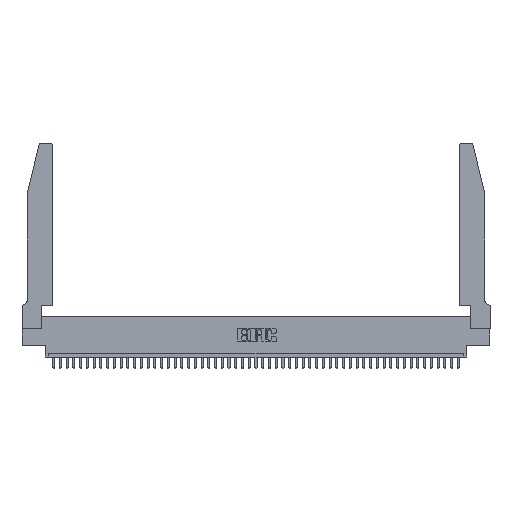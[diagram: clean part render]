
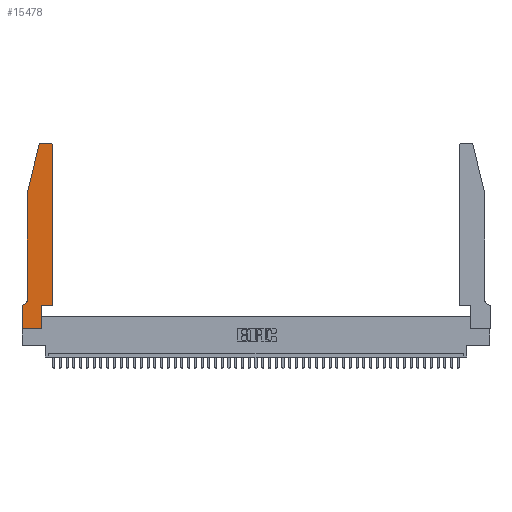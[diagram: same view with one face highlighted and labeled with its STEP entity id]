
A CAD part, top view. The second image highlights one B-rep face of the part: STEP entity #15478.
In plain terms, the highlighted planar face has unit normal (0, 0, 1).
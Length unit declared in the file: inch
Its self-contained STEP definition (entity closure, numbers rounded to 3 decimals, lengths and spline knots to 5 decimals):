
#88 = ORIENTED_EDGE ( 'NONE', *, *, #6962, .T. ) ;
#566 = CARTESIAN_POINT ( 'NONE',  ( 0., 0.35, 0.37 ) ) ;
#2548 = LINE ( 'NONE', #25278, #21240 ) ;
#2720 = DIRECTION ( 'NONE',  ( 0., 1., 0. ) ) ;
#3032 = VERTEX_POINT ( 'NONE', #42232 ) ;
#3805 = AXIS2_PLACEMENT_3D ( 'NONE', #36705, #41069, #40446 ) ;
#4126 = LINE ( 'NONE', #10552, #36232 ) ;
#6044 = VECTOR ( 'NONE', #23524, 39.37008 ) ;
#6074 = VERTEX_POINT ( 'NONE', #7845 ) ;
#6962 = EDGE_CURVE ( 'NONE', #32405, #3032, #40189, .T. ) ;
#7144 = CARTESIAN_POINT ( 'NONE',  ( 0.0055, 0.42, 0.37 ) ) ;
#7160 = EDGE_CURVE ( 'NONE', #43661, #17790, #11598, .T. ) ;
#7193 = LINE ( 'NONE', #15904, #6044 ) ;
#7311 = CARTESIAN_POINT ( 'NONE',  ( 0.2605, 2.75, 0.37 ) ) ;
#7845 = CARTESIAN_POINT ( 'NONE',  ( 0.2865, 0., 0.37 ) ) ;
#8034 = CIRCLE ( 'NONE', #22942, 0.03 ) ;
#9310 = DIRECTION ( 'NONE',  ( -1., 0., 0. ) ) ;
#9410 = VECTOR ( 'NONE', #21468, 39.37008 ) ;
#9710 = CARTESIAN_POINT ( 'NONE',  ( 0., 0.35, 0.37 ) ) ;
#10404 = ORIENTED_EDGE ( 'NONE', *, *, #36614, .T. ) ;
#10552 = CARTESIAN_POINT ( 'NONE',  ( 0.0755, 2., 0.37 ) ) ;
#10879 = DIRECTION ( 'NONE',  ( -1., 0., 0. ) ) ;
#11598 = LINE ( 'NONE', #15957, #30310 ) ;
#11695 = CIRCLE ( 'NONE', #18827, 0.07 ) ;
#13011 = EDGE_CURVE ( 'NONE', #21215, #30561, #38854, .T. ) ;
#13251 = LINE ( 'NONE', #7311, #25518 ) ;
#14350 = DIRECTION ( 'NONE',  ( 0., 0., -1. ) ) ;
#14723 = VERTEX_POINT ( 'NONE', #16777 ) ;
#14812 = VERTEX_POINT ( 'NONE', #39039 ) ;
#15478 = ADVANCED_FACE ( 'NONE', ( #28745 ), #26694, .T. ) ;
#15545 = CARTESIAN_POINT ( 'NONE',  ( 0., 0., 0.37 ) ) ;
#15624 = VECTOR ( 'NONE', #9310, 39.37008 ) ;
#15684 = ORIENTED_EDGE ( 'NONE', *, *, #27631, .T. ) ;
#15904 = CARTESIAN_POINT ( 'NONE',  ( 0., 0., 0.37 ) ) ;
#15957 = CARTESIAN_POINT ( 'NONE',  ( 0.4505, 0.35, 0.37 ) ) ;
#16777 = CARTESIAN_POINT ( 'NONE',  ( 0.284, 2.75, 0.37 ) ) ;
#17431 = CARTESIAN_POINT ( 'NONE',  ( 0.4505, 0.35, 0.37 ) ) ;
#17790 = VERTEX_POINT ( 'NONE', #17431 ) ;
#18008 = DIRECTION ( 'NONE',  ( 0., 0., 1. ) ) ;
#18670 = ORIENTED_EDGE ( 'NONE', *, *, #43840, .T. ) ;
#18827 = AXIS2_PLACEMENT_3D ( 'NONE', #7144, #14350, #10879 ) ;
#19296 = LINE ( 'NONE', #43368, #9410 ) ;
#19602 = ORIENTED_EDGE ( 'NONE', *, *, #7160, .T. ) ;
#20277 = VERTEX_POINT ( 'NONE', #28497 ) ;
#20311 = VECTOR ( 'NONE', #39492, 39.37008 ) ;
#21215 = VERTEX_POINT ( 'NONE', #9710 ) ;
#21240 = VECTOR ( 'NONE', #2720, 39.37008 ) ;
#21468 = DIRECTION ( 'NONE',  ( 0., 1., 0. ) ) ;
#21823 = ORIENTED_EDGE ( 'NONE', *, *, #35399, .T. ) ;
#21848 = ORIENTED_EDGE ( 'NONE', *, *, #22496, .T. ) ;
#22496 = EDGE_CURVE ( 'NONE', #6074, #43661, #19296, .T. ) ;
#22669 = ORIENTED_EDGE ( 'NONE', *, *, #40608, .T. ) ;
#22921 = DIRECTION ( 'NONE',  ( 1., 0., 0. ) ) ;
#22942 = AXIS2_PLACEMENT_3D ( 'NONE', #32560, #18008, #44121 ) ;
#23524 = DIRECTION ( 'NONE',  ( 1., 0., 0. ) ) ;
#24866 = CARTESIAN_POINT ( 'NONE',  ( 0.0755, 0.42, 0.37 ) ) ;
#25278 = CARTESIAN_POINT ( 'NONE',  ( 0.4505, 0.35, 0.37 ) ) ;
#25518 = VECTOR ( 'NONE', #44655, 39.37008 ) ;
#25780 = VERTEX_POINT ( 'NONE', #24866 ) ;
#26415 = ORIENTED_EDGE ( 'NONE', *, *, #13011, .T. ) ;
#26441 = CARTESIAN_POINT ( 'NONE',  ( 0.0055, 0.35, 0.37 ) ) ;
#26443 = DIRECTION ( 'NONE',  ( 0., -1., 0. ) ) ;
#26694 = PLANE ( 'NONE',  #39971 ) ;
#27224 = ORIENTED_EDGE ( 'NONE', *, *, #38644, .T. ) ;
#27432 = CARTESIAN_POINT ( 'NONE',  ( 0.0755, 0.35, 0.37 ) ) ;
#27631 = EDGE_CURVE ( 'NONE', #25780, #32143, #11695, .T. ) ;
#28424 = CARTESIAN_POINT ( 'NONE',  ( 0.25487, 2.72718, 0.37 ) ) ;
#28497 = CARTESIAN_POINT ( 'NONE',  ( 0.4505, 2.72, 0.37 ) ) ;
#28745 = FACE_OUTER_BOUND ( 'NONE', #44718, .T. ) ;
#30133 = DIRECTION ( 'NONE',  ( 1., 0., 0. ) ) ;
#30310 = VECTOR ( 'NONE', #22921, 39.37008 ) ;
#30561 = VERTEX_POINT ( 'NONE', #37762 ) ;
#30996 = EDGE_CURVE ( 'NONE', #20277, #14812, #8034, .T. ) ;
#31943 = CIRCLE ( 'NONE', #3805, 0.03 ) ;
#32143 = VERTEX_POINT ( 'NONE', #26441 ) ;
#32405 = VERTEX_POINT ( 'NONE', #28424 ) ;
#32560 = CARTESIAN_POINT ( 'NONE',  ( 0.4205, 2.72, 0.37 ) ) ;
#34161 = VECTOR ( 'NONE', #26443, 39.37008 ) ;
#35399 = EDGE_CURVE ( 'NONE', #32143, #21215, #35485, .T. ) ;
#35485 = LINE ( 'NONE', #27432, #15624 ) ;
#35905 = CARTESIAN_POINT ( 'NONE',  ( 0.0755, 2., 0.37 ) ) ;
#36232 = VECTOR ( 'NONE', #48362, 39.37008 ) ;
#36260 = ORIENTED_EDGE ( 'NONE', *, *, #30996, .T. ) ;
#36614 = EDGE_CURVE ( 'NONE', #17790, #20277, #2548, .T. ) ;
#36705 = CARTESIAN_POINT ( 'NONE',  ( 0.284, 2.72, 0.37 ) ) ;
#37762 = CARTESIAN_POINT ( 'NONE',  ( 0., 0., 0.37 ) ) ;
#38644 = EDGE_CURVE ( 'NONE', #3032, #25780, #4126, .T. ) ;
#38854 = LINE ( 'NONE', #15545, #34161 ) ;
#39039 = CARTESIAN_POINT ( 'NONE',  ( 0.4205, 2.75, 0.37 ) ) ;
#39492 = DIRECTION ( 'NONE',  ( -0.239, -0.971, 0. ) ) ;
#39971 = AXIS2_PLACEMENT_3D ( 'NONE', #566, #41860, #30133 ) ;
#40189 = LINE ( 'NONE', #35905, #20311 ) ;
#40446 = DIRECTION ( 'NONE',  ( 1., 0., 0. ) ) ;
#40608 = EDGE_CURVE ( 'NONE', #30561, #6074, #7193, .T. ) ;
#41069 = DIRECTION ( 'NONE',  ( 0., 0., 1. ) ) ;
#41860 = DIRECTION ( 'NONE',  ( 0., 0., 1. ) ) ;
#42232 = CARTESIAN_POINT ( 'NONE',  ( 0.0755, 2., 0.37 ) ) ;
#43368 = CARTESIAN_POINT ( 'NONE',  ( 0.2865, 0.35, 0.37 ) ) ;
#43661 = VERTEX_POINT ( 'NONE', #43723 ) ;
#43723 = CARTESIAN_POINT ( 'NONE',  ( 0.2865, 0.35, 0.37 ) ) ;
#43840 = EDGE_CURVE ( 'NONE', #14812, #14723, #13251, .T. ) ;
#43852 = EDGE_CURVE ( 'NONE', #14723, #32405, #31943, .T. ) ;
#44121 = DIRECTION ( 'NONE',  ( 1., 0., 0. ) ) ;
#44655 = DIRECTION ( 'NONE',  ( -1., 0., 0. ) ) ;
#44718 = EDGE_LOOP ( 'NONE', ( #18670, #47516, #88, #27224, #15684, #21823, #26415, #22669, #21848, #19602, #10404, #36260 ) ) ;
#47516 = ORIENTED_EDGE ( 'NONE', *, *, #43852, .T. ) ;
#48362 = DIRECTION ( 'NONE',  ( 0., -1., 0. ) ) ;
